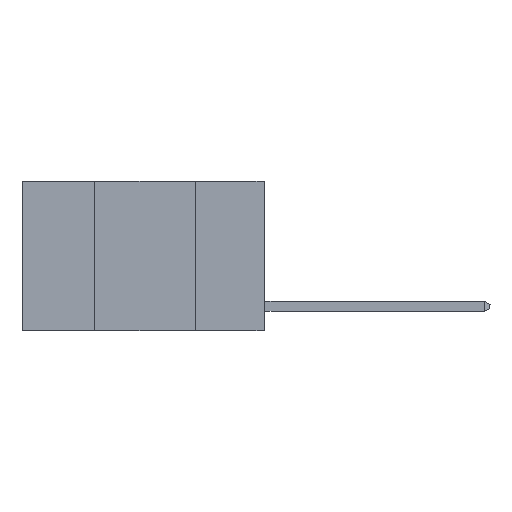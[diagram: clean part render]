
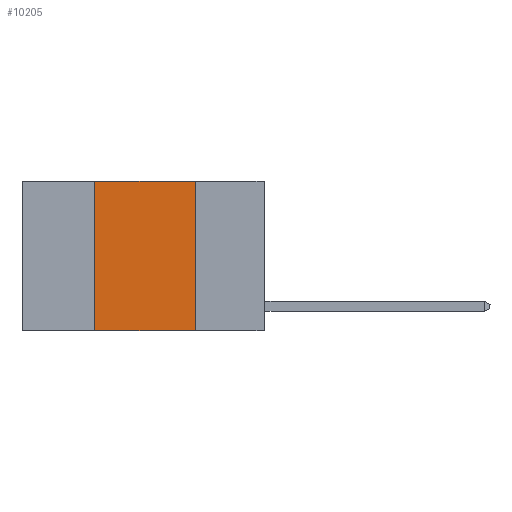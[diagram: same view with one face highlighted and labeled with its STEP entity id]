
A CAD part, left-side view. The second image highlights one B-rep face of the part: STEP entity #10205.
In plain terms, the highlighted planar face has unit normal (-1, 0, 0).
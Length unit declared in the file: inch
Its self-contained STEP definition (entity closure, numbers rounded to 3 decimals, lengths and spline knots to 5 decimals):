
#518 = EDGE_CURVE ( 'NONE', #11770, #8576, #12901, .T. ) ;
#688 = VECTOR ( 'NONE', #13256, 39.37008 ) ;
#1248 = ORIENTED_EDGE ( 'NONE', *, *, #1346, .T. ) ;
#1346 = EDGE_CURVE ( 'NONE', #11770, #1974, #13434, .T. ) ;
#1891 = ORIENTED_EDGE ( 'NONE', *, *, #2484, .F. ) ;
#1974 = VERTEX_POINT ( 'NONE', #4427 ) ;
#2096 = EDGE_CURVE ( 'NONE', #7048, #1974, #12503, .T. ) ;
#2484 = EDGE_CURVE ( 'NONE', #8576, #7048, #11860, .T. ) ;
#2496 = DIRECTION ( 'NONE',  ( 0., 0., 1. ) ) ;
#2604 = DIRECTION ( 'NONE',  ( 0., 0., -1. ) ) ;
#4427 = CARTESIAN_POINT ( 'NONE',  ( 0., 0.17, -0.37 ) ) ;
#4994 = ORIENTED_EDGE ( 'NONE', *, *, #518, .F. ) ;
#5121 = ORIENTED_EDGE ( 'NONE', *, *, #2096, .F. ) ;
#6790 = VECTOR ( 'NONE', #7687, 39.37008 ) ;
#7004 = CARTESIAN_POINT ( 'NONE',  ( 0., 0.42, 0. ) ) ;
#7048 = VERTEX_POINT ( 'NONE', #9686 ) ;
#7096 = CARTESIAN_POINT ( 'NONE',  ( 0., 0.6, 0. ) ) ;
#7687 = DIRECTION ( 'NONE',  ( 0., -1., 0. ) ) ;
#7826 = VECTOR ( 'NONE', #10622, 39.37008 ) ;
#8576 = VERTEX_POINT ( 'NONE', #9041 ) ;
#9041 = CARTESIAN_POINT ( 'NONE',  ( 0., 0.42, 0. ) ) ;
#9134 = AXIS2_PLACEMENT_3D ( 'NONE', #7096, #9336, #2604 ) ;
#9336 = DIRECTION ( 'NONE',  ( 1., 0., 0. ) ) ;
#9535 = CARTESIAN_POINT ( 'NONE',  ( 0., 0.6, -0.37 ) ) ;
#9602 = EDGE_LOOP ( 'NONE', ( #5121, #1891, #4994, #1248 ) ) ;
#9686 = CARTESIAN_POINT ( 'NONE',  ( 0., 0.17, 0. ) ) ;
#10205 = ADVANCED_FACE ( 'NONE', ( #11576 ), #12451, .F. ) ;
#10622 = DIRECTION ( 'NONE',  ( 0., -1., 0. ) ) ;
#11576 = FACE_OUTER_BOUND ( 'NONE', #9602, .T. ) ;
#11770 = VERTEX_POINT ( 'NONE', #13735 ) ;
#11860 = LINE ( 'NONE', #13970, #6790 ) ;
#12451 = PLANE ( 'NONE',  #9134 ) ;
#12503 = LINE ( 'NONE', #13212, #688 ) ;
#12594 = VECTOR ( 'NONE', #2496, 39.37008 ) ;
#12901 = LINE ( 'NONE', #7004, #12594 ) ;
#13212 = CARTESIAN_POINT ( 'NONE',  ( 0., 0.17, 0. ) ) ;
#13256 = DIRECTION ( 'NONE',  ( 0., 0., -1. ) ) ;
#13434 = LINE ( 'NONE', #9535, #7826 ) ;
#13735 = CARTESIAN_POINT ( 'NONE',  ( 0., 0.42, -0.37 ) ) ;
#13970 = CARTESIAN_POINT ( 'NONE',  ( 0., 0.6, 0. ) ) ;
